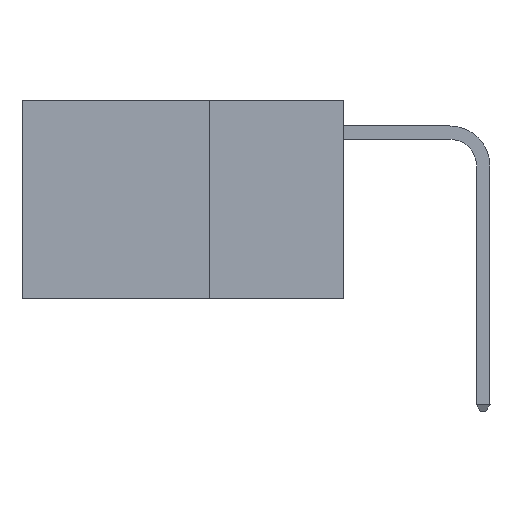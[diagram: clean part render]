
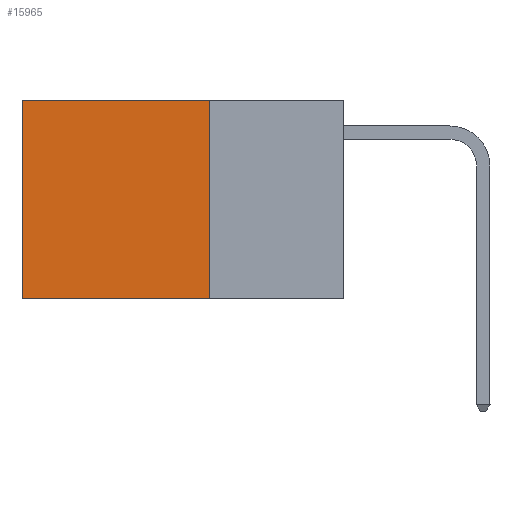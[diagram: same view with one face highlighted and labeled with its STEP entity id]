
A CAD part, left-side view. The second image highlights one B-rep face of the part: STEP entity #15965.
In plain terms, the highlighted planar face has unit normal (-1, 0, 0).
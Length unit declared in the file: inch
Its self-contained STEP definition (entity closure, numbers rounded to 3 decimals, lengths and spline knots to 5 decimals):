
#565 = EDGE_LOOP ( 'NONE', ( #9165, #12224, #1556, #10998 ) ) ;
#1277 = EDGE_CURVE ( 'NONE', #9625, #11137, #11205, .T. ) ;
#1556 = ORIENTED_EDGE ( 'NONE', *, *, #7750, .F. ) ;
#1604 = CARTESIAN_POINT ( 'NONE',  ( 0.2625, 0.25, 0. ) ) ;
#1868 = CARTESIAN_POINT ( 'NONE',  ( 0.2625, 0.25, 0. ) ) ;
#2525 = LINE ( 'NONE', #13297, #12456 ) ;
#3170 = DIRECTION ( 'NONE',  ( 0., 0., -1. ) ) ;
#3237 = CARTESIAN_POINT ( 'NONE',  ( 0.2625, 0.6, 0. ) ) ;
#4159 = VERTEX_POINT ( 'NONE', #4682 ) ;
#4243 = DIRECTION ( 'NONE',  ( 0., 1., 0. ) ) ;
#4682 = CARTESIAN_POINT ( 'NONE',  ( 0.2625, 0.25, 0. ) ) ;
#5916 = CARTESIAN_POINT ( 'NONE',  ( 0.2625, 0.25, -0.37 ) ) ;
#6455 = CARTESIAN_POINT ( 'NONE',  ( 0.2625, 0.6, -0.37 ) ) ;
#7291 = DIRECTION ( 'NONE',  ( 0., 0., -1. ) ) ;
#7750 = EDGE_CURVE ( 'NONE', #4159, #10960, #13381, .T. ) ;
#9165 = ORIENTED_EDGE ( 'NONE', *, *, #1277, .T. ) ;
#9357 = VECTOR ( 'NONE', #7291, 39.37008 ) ;
#9625 = VERTEX_POINT ( 'NONE', #3237 ) ;
#10960 = VERTEX_POINT ( 'NONE', #5916 ) ;
#10972 = DIRECTION ( 'NONE',  ( 1., 0., 0. ) ) ;
#10998 = ORIENTED_EDGE ( 'NONE', *, *, #12637, .T. ) ;
#11017 = VECTOR ( 'NONE', #16007, 39.37008 ) ;
#11137 = VERTEX_POINT ( 'NONE', #6455 ) ;
#11205 = LINE ( 'NONE', #16243, #9357 ) ;
#11746 = LINE ( 'NONE', #16185, #11017 ) ;
#12224 = ORIENTED_EDGE ( 'NONE', *, *, #15828, .F. ) ;
#12257 = DIRECTION ( 'NONE',  ( 0., 0., -1. ) ) ;
#12456 = VECTOR ( 'NONE', #4243, 39.37008 ) ;
#12637 = EDGE_CURVE ( 'NONE', #4159, #9625, #11746, .T. ) ;
#13297 = CARTESIAN_POINT ( 'NONE',  ( 0.2625, 0.25, -0.37 ) ) ;
#13381 = LINE ( 'NONE', #1604, #13732 ) ;
#13732 = VECTOR ( 'NONE', #12257, 39.37008 ) ;
#13839 = FACE_OUTER_BOUND ( 'NONE', #565, .T. ) ;
#15828 = EDGE_CURVE ( 'NONE', #10960, #11137, #2525, .T. ) ;
#15941 = PLANE ( 'NONE',  #16110 ) ;
#15965 = ADVANCED_FACE ( 'NONE', ( #13839 ), #15941, .F. ) ;
#16007 = DIRECTION ( 'NONE',  ( 0., 1., 0. ) ) ;
#16110 = AXIS2_PLACEMENT_3D ( 'NONE', #1868, #10972, #3170 ) ;
#16185 = CARTESIAN_POINT ( 'NONE',  ( 0.2625, 0.25, 0. ) ) ;
#16243 = CARTESIAN_POINT ( 'NONE',  ( 0.2625, 0.6, 0. ) ) ;
